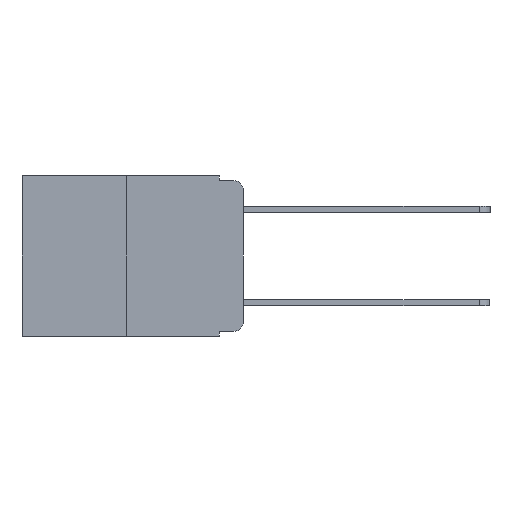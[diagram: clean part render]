
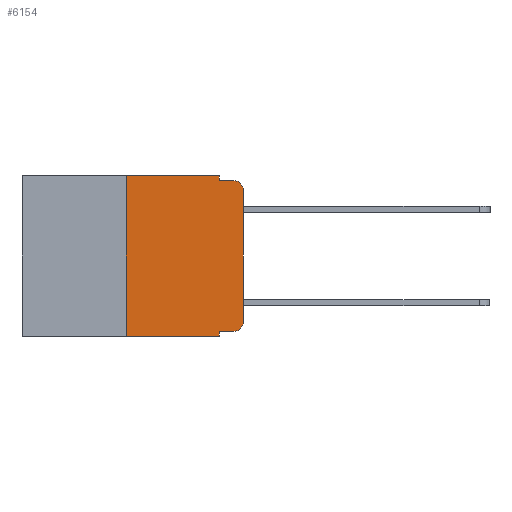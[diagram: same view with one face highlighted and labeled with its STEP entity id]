
A CAD part, left-side view. The second image highlights one B-rep face of the part: STEP entity #6154.
In plain terms, the highlighted planar face has unit normal (-1, 0, 0).
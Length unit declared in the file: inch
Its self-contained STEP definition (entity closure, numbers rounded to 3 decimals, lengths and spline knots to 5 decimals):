
#165 = ORIENTED_EDGE ( 'NONE', *, *, #8041, .F. ) ;
#286 = CARTESIAN_POINT ( 'NONE',  ( 0., 0., 0. ) ) ;
#329 = ORIENTED_EDGE ( 'NONE', *, *, #4081, .F. ) ;
#338 = CARTESIAN_POINT ( 'NONE',  ( 0., 0., -0.03 ) ) ;
#407 = VECTOR ( 'NONE', #4858, 39.37008 ) ;
#435 = FACE_OUTER_BOUND ( 'NONE', #3662, .T. ) ;
#723 = PLANE ( 'NONE',  #3458 ) ;
#792 = ORIENTED_EDGE ( 'NONE', *, *, #8344, .T. ) ;
#794 = CARTESIAN_POINT ( 'NONE',  ( 0., 0.051, -0.343 ) ) ;
#1044 = CARTESIAN_POINT ( 'NONE',  ( 0., 0.25, 0. ) ) ;
#1060 = ORIENTED_EDGE ( 'NONE', *, *, #4340, .F. ) ;
#1107 = ORIENTED_EDGE ( 'NONE', *, *, #2988, .T. ) ;
#1401 = VERTEX_POINT ( 'NONE', #7811 ) ;
#1674 = VERTEX_POINT ( 'NONE', #10115 ) ;
#1709 = VERTEX_POINT ( 'NONE', #7636 ) ;
#1784 = VERTEX_POINT ( 'NONE', #10001 ) ;
#1787 = DIRECTION ( 'NONE',  ( 0., 0., -1. ) ) ;
#2294 = VECTOR ( 'NONE', #1787, 39.37008 ) ;
#2335 = ORIENTED_EDGE ( 'NONE', *, *, #9274, .F. ) ;
#2639 = VECTOR ( 'NONE', #4952, 39.37008 ) ;
#2641 = AXIS2_PLACEMENT_3D ( 'NONE', #9410, #9323, #9387 ) ;
#2658 = VECTOR ( 'NONE', #3214, 39.37008 ) ;
#2789 = CARTESIAN_POINT ( 'NONE',  ( 0., 0.051, 0. ) ) ;
#2931 = LINE ( 'NONE', #6598, #2639 ) ;
#2938 = CIRCLE ( 'NONE', #5635, 0.02 ) ;
#2988 = EDGE_CURVE ( 'NONE', #10443, #9453, #9251, .T. ) ;
#2992 = VERTEX_POINT ( 'NONE', #6442 ) ;
#3214 = DIRECTION ( 'NONE',  ( 0., 0., 1. ) ) ;
#3248 = EDGE_CURVE ( 'NONE', #1784, #6016, #5469, .T. ) ;
#3318 = CARTESIAN_POINT ( 'NONE',  ( 0., 0.02, -0.03 ) ) ;
#3320 = VERTEX_POINT ( 'NONE', #338 ) ;
#3458 = AXIS2_PLACEMENT_3D ( 'NONE', #5403, #8500, #3682 ) ;
#3662 = EDGE_LOOP ( 'NONE', ( #9842, #8010, #2335, #165, #329, #6221, #1107, #1060, #792, #5188 ) ) ;
#3682 = DIRECTION ( 'NONE',  ( 0., 0., -1. ) ) ;
#4081 = EDGE_CURVE ( 'NONE', #6156, #1674, #2931, .T. ) ;
#4260 = DIRECTION ( 'NONE',  ( 0., 0., -1. ) ) ;
#4340 = EDGE_CURVE ( 'NONE', #1709, #9453, #5306, .T. ) ;
#4713 = EDGE_CURVE ( 'NONE', #10443, #6156, #7682, .T. ) ;
#4858 = DIRECTION ( 'NONE',  ( 0., -1., 0. ) ) ;
#4952 = DIRECTION ( 'NONE',  ( 0., -1., 0. ) ) ;
#5049 = VECTOR ( 'NONE', #8940, 39.37008 ) ;
#5188 = ORIENTED_EDGE ( 'NONE', *, *, #3248, .T. ) ;
#5298 = CARTESIAN_POINT ( 'NONE',  ( 0., 0., -0.313 ) ) ;
#5300 = EDGE_CURVE ( 'NONE', #6016, #3320, #10457, .T. ) ;
#5306 = LINE ( 'NONE', #8241, #5049 ) ;
#5403 = CARTESIAN_POINT ( 'NONE',  ( 0., 0.473, 0. ) ) ;
#5416 = LINE ( 'NONE', #7255, #407 ) ;
#5424 = CARTESIAN_POINT ( 'NONE',  ( 0., 0.051, -0.01 ) ) ;
#5469 = CIRCLE ( 'NONE', #2641, 0.02 ) ;
#5635 = AXIS2_PLACEMENT_3D ( 'NONE', #3318, #8929, #4260 ) ;
#5895 = EDGE_CURVE ( 'NONE', #3320, #2992, #2938, .T. ) ;
#6016 = VERTEX_POINT ( 'NONE', #5298 ) ;
#6154 = ADVANCED_FACE ( 'NONE', ( #435 ), #723, .F. ) ;
#6156 = VERTEX_POINT ( 'NONE', #7777 ) ;
#6169 = VECTOR ( 'NONE', #10476, 39.37008 ) ;
#6221 = ORIENTED_EDGE ( 'NONE', *, *, #4713, .F. ) ;
#6442 = CARTESIAN_POINT ( 'NONE',  ( 0., 0.02, -0.01 ) ) ;
#6568 = CARTESIAN_POINT ( 'NONE',  ( 0., 0.25, -0.343 ) ) ;
#6598 = CARTESIAN_POINT ( 'NONE',  ( 0., 0.473, 0. ) ) ;
#7255 = CARTESIAN_POINT ( 'NONE',  ( 0., 0.051, -0.333 ) ) ;
#7261 = DIRECTION ( 'NONE',  ( 0., 0., 1. ) ) ;
#7361 = VECTOR ( 'NONE', #9473, 39.37008 ) ;
#7636 = CARTESIAN_POINT ( 'NONE',  ( 0., 0.051, -0.333 ) ) ;
#7682 = LINE ( 'NONE', #1044, #9544 ) ;
#7777 = CARTESIAN_POINT ( 'NONE',  ( 0., 0.25, 0. ) ) ;
#7811 = CARTESIAN_POINT ( 'NONE',  ( 0., 0.051, -0.01 ) ) ;
#8010 = ORIENTED_EDGE ( 'NONE', *, *, #5895, .T. ) ;
#8041 = EDGE_CURVE ( 'NONE', #1674, #1401, #8874, .T. ) ;
#8209 = LINE ( 'NONE', #5424, #6169 ) ;
#8241 = CARTESIAN_POINT ( 'NONE',  ( 0., 0.051, 0. ) ) ;
#8344 = EDGE_CURVE ( 'NONE', #1709, #1784, #5416, .T. ) ;
#8500 = DIRECTION ( 'NONE',  ( 1., 0., 0. ) ) ;
#8874 = LINE ( 'NONE', #2789, #2294 ) ;
#8929 = DIRECTION ( 'NONE',  ( -1., 0., 0. ) ) ;
#8940 = DIRECTION ( 'NONE',  ( 0., 0., -1. ) ) ;
#9251 = LINE ( 'NONE', #9455, #7361 ) ;
#9274 = EDGE_CURVE ( 'NONE', #1401, #2992, #8209, .T. ) ;
#9323 = DIRECTION ( 'NONE',  ( -1., 0., 0. ) ) ;
#9387 = DIRECTION ( 'NONE',  ( 0., 0., -1. ) ) ;
#9410 = CARTESIAN_POINT ( 'NONE',  ( 0., 0.02, -0.313 ) ) ;
#9453 = VERTEX_POINT ( 'NONE', #794 ) ;
#9455 = CARTESIAN_POINT ( 'NONE',  ( 0., 0.473, -0.343 ) ) ;
#9473 = DIRECTION ( 'NONE',  ( 0., -1., 0. ) ) ;
#9544 = VECTOR ( 'NONE', #7261, 39.37008 ) ;
#9842 = ORIENTED_EDGE ( 'NONE', *, *, #5300, .T. ) ;
#10001 = CARTESIAN_POINT ( 'NONE',  ( 0., 0.02, -0.333 ) ) ;
#10115 = CARTESIAN_POINT ( 'NONE',  ( 0., 0.051, 0. ) ) ;
#10443 = VERTEX_POINT ( 'NONE', #6568 ) ;
#10457 = LINE ( 'NONE', #286, #2658 ) ;
#10476 = DIRECTION ( 'NONE',  ( 0., -1., 0. ) ) ;
